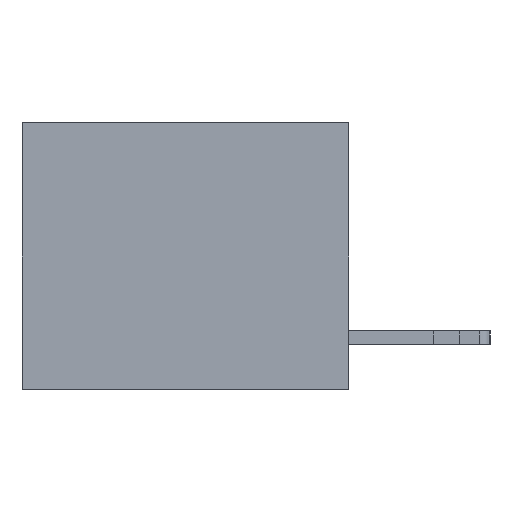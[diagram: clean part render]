
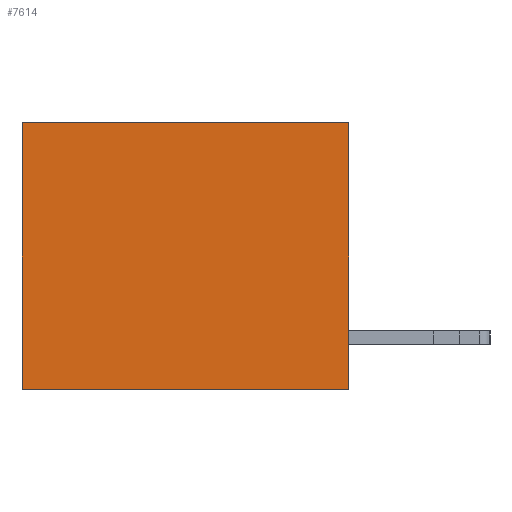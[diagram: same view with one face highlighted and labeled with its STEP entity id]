
A CAD part, left-side view. The second image highlights one B-rep face of the part: STEP entity #7614.
In plain terms, the highlighted planar face has unit normal (-1, 0, 0).
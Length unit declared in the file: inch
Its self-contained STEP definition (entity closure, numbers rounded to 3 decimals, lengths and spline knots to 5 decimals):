
#236 = CARTESIAN_POINT ( 'NONE',  ( 0.3165, 0., -0.49 ) ) ;
#620 = VECTOR ( 'NONE', #10960, 39.37008 ) ;
#785 = VERTEX_POINT ( 'NONE', #14127 ) ;
#838 = EDGE_CURVE ( 'NONE', #11366, #785, #12899, .T. ) ;
#1171 = DIRECTION ( 'NONE',  ( 1., 0., 0. ) ) ;
#1249 = EDGE_CURVE ( 'NONE', #785, #6442, #15094, .T. ) ;
#1650 = CARTESIAN_POINT ( 'NONE',  ( 0.3165, 0.6, -0.49 ) ) ;
#4350 = DIRECTION ( 'NONE',  ( 0., 0., -1. ) ) ;
#4395 = CARTESIAN_POINT ( 'NONE',  ( 0.3165, 0.6, 0. ) ) ;
#4736 = VECTOR ( 'NONE', #6574, 39.37008 ) ;
#5367 = ORIENTED_EDGE ( 'NONE', *, *, #1249, .F. ) ;
#5386 = CARTESIAN_POINT ( 'NONE',  ( 0.3165, 0.6, -0.49 ) ) ;
#6442 = VERTEX_POINT ( 'NONE', #5386 ) ;
#6534 = CARTESIAN_POINT ( 'NONE',  ( 0.3165, 0., -0.49 ) ) ;
#6574 = DIRECTION ( 'NONE',  ( 0., 0., -1. ) ) ;
#7030 = EDGE_CURVE ( 'NONE', #11366, #10113, #13040, .T. ) ;
#7570 = DIRECTION ( 'NONE',  ( 0., 0., -1. ) ) ;
#7614 = ADVANCED_FACE ( 'NONE', ( #18143 ), #13417, .F. ) ;
#8249 = VECTOR ( 'NONE', #8679, 39.37008 ) ;
#8679 = DIRECTION ( 'NONE',  ( 0., 1., 0. ) ) ;
#9475 = ORIENTED_EDGE ( 'NONE', *, *, #11664, .T. ) ;
#10113 = VERTEX_POINT ( 'NONE', #4395 ) ;
#10880 = EDGE_LOOP ( 'NONE', ( #9475, #5367, #19979, #19503 ) ) ;
#10960 = DIRECTION ( 'NONE',  ( 0., 1., 0. ) ) ;
#11366 = VERTEX_POINT ( 'NONE', #15455 ) ;
#11475 = LINE ( 'NONE', #1650, #19250 ) ;
#11638 = CARTESIAN_POINT ( 'NONE',  ( 0.3165, 0., 0. ) ) ;
#11664 = EDGE_CURVE ( 'NONE', #10113, #6442, #11475, .T. ) ;
#12008 = CARTESIAN_POINT ( 'NONE',  ( 0.3165, 0., -0.49 ) ) ;
#12899 = LINE ( 'NONE', #236, #4736 ) ;
#13040 = LINE ( 'NONE', #11638, #8249 ) ;
#13417 = PLANE ( 'NONE',  #15888 ) ;
#14127 = CARTESIAN_POINT ( 'NONE',  ( 0.3165, 0., -0.49 ) ) ;
#15094 = LINE ( 'NONE', #6534, #620 ) ;
#15455 = CARTESIAN_POINT ( 'NONE',  ( 0.3165, 0., 0. ) ) ;
#15888 = AXIS2_PLACEMENT_3D ( 'NONE', #12008, #1171, #4350 ) ;
#18143 = FACE_OUTER_BOUND ( 'NONE', #10880, .T. ) ;
#19250 = VECTOR ( 'NONE', #7570, 39.37008 ) ;
#19503 = ORIENTED_EDGE ( 'NONE', *, *, #7030, .T. ) ;
#19979 = ORIENTED_EDGE ( 'NONE', *, *, #838, .F. ) ;
